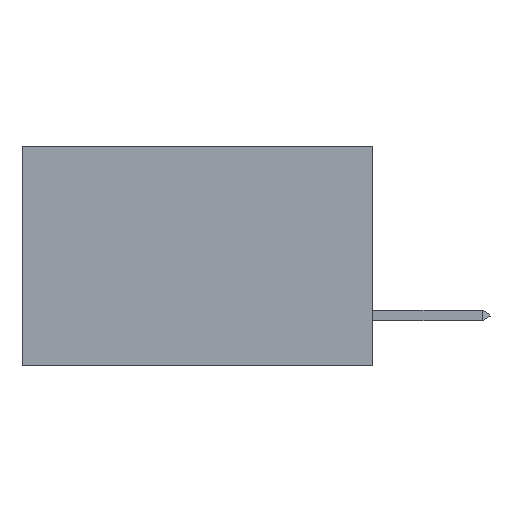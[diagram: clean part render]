
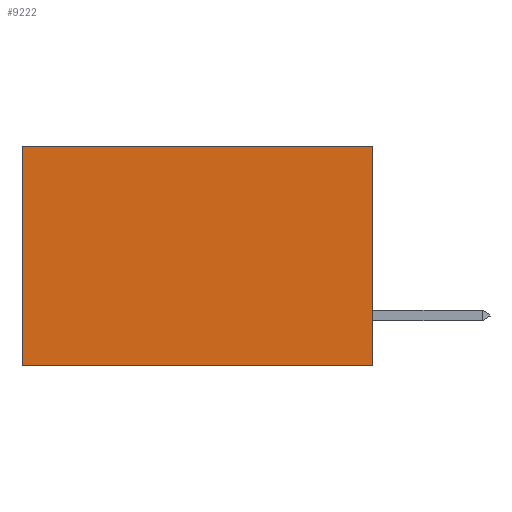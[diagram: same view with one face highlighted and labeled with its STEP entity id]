
A CAD part, left-side view. The second image highlights one B-rep face of the part: STEP entity #9222.
In plain terms, the highlighted planar face has unit normal (-1, 0, 0).
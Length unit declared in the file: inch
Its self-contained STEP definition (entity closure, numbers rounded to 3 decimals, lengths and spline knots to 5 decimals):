
#81 = EDGE_CURVE ( 'NONE', #10416, #12452, #6625, .T. ) ;
#105 = EDGE_CURVE ( 'NONE', #1350, #10416, #8643, .T. ) ;
#907 = EDGE_CURVE ( 'NONE', #3054, #12452, #11964, .T. ) ;
#1350 = VERTEX_POINT ( 'NONE', #11783 ) ;
#1460 = CARTESIAN_POINT ( 'NONE',  ( 0.277, 0., 0. ) ) ;
#1538 = CARTESIAN_POINT ( 'NONE',  ( 0.277, 0., -0.37 ) ) ;
#2050 = EDGE_CURVE ( 'NONE', #1350, #3054, #4383, .T. ) ;
#2619 = EDGE_LOOP ( 'NONE', ( #9141, #8711, #5999, #12490 ) ) ;
#3054 = VERTEX_POINT ( 'NONE', #12721 ) ;
#3679 = DIRECTION ( 'NONE',  ( 0., 0., -1. ) ) ;
#3965 = DIRECTION ( 'NONE',  ( 0., 1., 0. ) ) ;
#4383 = LINE ( 'NONE', #1460, #9612 ) ;
#4716 = AXIS2_PLACEMENT_3D ( 'NONE', #1538, #12059, #6345 ) ;
#4726 = FACE_OUTER_BOUND ( 'NONE', #2619, .T. ) ;
#5166 = PLANE ( 'NONE',  #4716 ) ;
#5514 = CARTESIAN_POINT ( 'NONE',  ( 0.277, 0.59, -0.37 ) ) ;
#5713 = DIRECTION ( 'NONE',  ( 0., 1., 0. ) ) ;
#5920 = VECTOR ( 'NONE', #3679, 39.37008 ) ;
#5999 = ORIENTED_EDGE ( 'NONE', *, *, #105, .F. ) ;
#6345 = DIRECTION ( 'NONE',  ( 0., 0., -1. ) ) ;
#6625 = LINE ( 'NONE', #7348, #6931 ) ;
#6931 = VECTOR ( 'NONE', #5713, 39.37008 ) ;
#7348 = CARTESIAN_POINT ( 'NONE',  ( 0.277, 0., -0.37 ) ) ;
#8643 = LINE ( 'NONE', #9186, #5920 ) ;
#8711 = ORIENTED_EDGE ( 'NONE', *, *, #81, .F. ) ;
#9141 = ORIENTED_EDGE ( 'NONE', *, *, #907, .T. ) ;
#9186 = CARTESIAN_POINT ( 'NONE',  ( 0.277, 0., -0.37 ) ) ;
#9222 = ADVANCED_FACE ( 'NONE', ( #4726 ), #5166, .F. ) ;
#9523 = VECTOR ( 'NONE', #10990, 39.37008 ) ;
#9612 = VECTOR ( 'NONE', #3965, 39.37008 ) ;
#10342 = CARTESIAN_POINT ( 'NONE',  ( 0.277, 0., -0.37 ) ) ;
#10416 = VERTEX_POINT ( 'NONE', #10342 ) ;
#10990 = DIRECTION ( 'NONE',  ( 0., 0., -1. ) ) ;
#11783 = CARTESIAN_POINT ( 'NONE',  ( 0.277, 0., 0. ) ) ;
#11964 = LINE ( 'NONE', #13584, #9523 ) ;
#12059 = DIRECTION ( 'NONE',  ( 1., 0., 0. ) ) ;
#12452 = VERTEX_POINT ( 'NONE', #5514 ) ;
#12490 = ORIENTED_EDGE ( 'NONE', *, *, #2050, .T. ) ;
#12721 = CARTESIAN_POINT ( 'NONE',  ( 0.277, 0.59, 0. ) ) ;
#13584 = CARTESIAN_POINT ( 'NONE',  ( 0.277, 0.59, -0.37 ) ) ;
